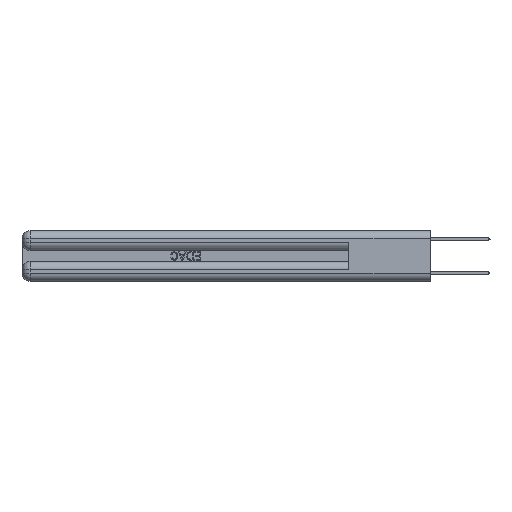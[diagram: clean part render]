
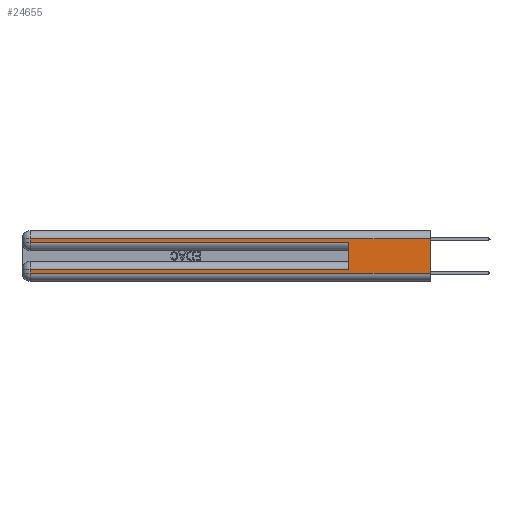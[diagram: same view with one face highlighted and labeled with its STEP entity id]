
A CAD part, left-side view. The second image highlights one B-rep face of the part: STEP entity #24655.
In plain terms, the highlighted planar face has unit normal (-1, 0, 0).
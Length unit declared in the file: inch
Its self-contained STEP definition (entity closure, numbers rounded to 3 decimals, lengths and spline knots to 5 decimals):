
#192 = DIRECTION ( 'NONE',  ( 0., 0., -1. ) ) ;
#230 = VERTEX_POINT ( 'NONE', #11451 ) ;
#247 = VERTEX_POINT ( 'NONE', #9179 ) ;
#296 = VECTOR ( 'NONE', #5717, 39.37008 ) ;
#312 = CARTESIAN_POINT ( 'NONE',  ( 0., 0.6, 0.285 ) ) ;
#361 = VERTEX_POINT ( 'NONE', #24869 ) ;
#596 = ORIENTED_EDGE ( 'NONE', *, *, #27372, .T. ) ;
#1087 = CARTESIAN_POINT ( 'NONE',  ( 0., 0.6, 0.145 ) ) ;
#1525 = CARTESIAN_POINT ( 'NONE',  ( 0., 2.94, 0.37 ) ) ;
#1733 = CARTESIAN_POINT ( 'NONE',  ( 0., 0., 0.06 ) ) ;
#2167 = CARTESIAN_POINT ( 'NONE',  ( 0., 2.94, 0.06 ) ) ;
#3639 = EDGE_CURVE ( 'NONE', #230, #12751, #26774, .T. ) ;
#4480 = PLANE ( 'NONE',  #22004 ) ;
#5116 = VERTEX_POINT ( 'NONE', #23936 ) ;
#5717 = DIRECTION ( 'NONE',  ( 0., 1., 0. ) ) ;
#5820 = LINE ( 'NONE', #12741, #21688 ) ;
#7189 = EDGE_CURVE ( 'NONE', #23041, #247, #27964, .T. ) ;
#8208 = DIRECTION ( 'NONE',  ( 0., -1., 0. ) ) ;
#8730 = CARTESIAN_POINT ( 'NONE',  ( 0., 2.94, 0.37 ) ) ;
#9179 = CARTESIAN_POINT ( 'NONE',  ( 0., 0., 0.06 ) ) ;
#9266 = CARTESIAN_POINT ( 'NONE',  ( 0., 0., 0.31 ) ) ;
#9878 = CARTESIAN_POINT ( 'NONE',  ( 0., 0., 0.085 ) ) ;
#10359 = ORIENTED_EDGE ( 'NONE', *, *, #12345, .F. ) ;
#11451 = CARTESIAN_POINT ( 'NONE',  ( 0., 0.6, 0.085 ) ) ;
#11720 = VERTEX_POINT ( 'NONE', #25460 ) ;
#11728 = LINE ( 'NONE', #9266, #27562 ) ;
#12126 = ORIENTED_EDGE ( 'NONE', *, *, #3639, .F. ) ;
#12345 = EDGE_CURVE ( 'NONE', #15269, #247, #18260, .T. ) ;
#12392 = DIRECTION ( 'NONE',  ( 0., 0., -1. ) ) ;
#12741 = CARTESIAN_POINT ( 'NONE',  ( 0., 0., 0.285 ) ) ;
#12751 = VERTEX_POINT ( 'NONE', #312 ) ;
#14152 = VECTOR ( 'NONE', #12392, 39.37008 ) ;
#14331 = VECTOR ( 'NONE', #18559, 39.37008 ) ;
#14810 = LINE ( 'NONE', #8730, #25882 ) ;
#14822 = DIRECTION ( 'NONE',  ( 0., 0., -1. ) ) ;
#15123 = DIRECTION ( 'NONE',  ( 0., 1., 0. ) ) ;
#15269 = VERTEX_POINT ( 'NONE', #18338 ) ;
#15449 = ORIENTED_EDGE ( 'NONE', *, *, #24988, .T. ) ;
#17200 = FACE_OUTER_BOUND ( 'NONE', #26297, .T. ) ;
#17418 = DIRECTION ( 'NONE',  ( 1., 0., 0. ) ) ;
#17863 = LINE ( 'NONE', #1525, #14152 ) ;
#17918 = ORIENTED_EDGE ( 'NONE', *, *, #7189, .T. ) ;
#18260 = LINE ( 'NONE', #27507, #23291 ) ;
#18338 = CARTESIAN_POINT ( 'NONE',  ( 0., 0., 0.31 ) ) ;
#18559 = DIRECTION ( 'NONE',  ( 0., 0., 1. ) ) ;
#18565 = LINE ( 'NONE', #9878, #296 ) ;
#18575 = EDGE_CURVE ( 'NONE', #11720, #12751, #5820, .T. ) ;
#20685 = DIRECTION ( 'NONE',  ( 0., -1., 0. ) ) ;
#21052 = ORIENTED_EDGE ( 'NONE', *, *, #18575, .T. ) ;
#21360 = ORIENTED_EDGE ( 'NONE', *, *, #24446, .T. ) ;
#21585 = ORIENTED_EDGE ( 'NONE', *, *, #27872, .T. ) ;
#21651 = DIRECTION ( 'NONE',  ( 0., 0., -1. ) ) ;
#21688 = VECTOR ( 'NONE', #8208, 39.37008 ) ;
#22004 = AXIS2_PLACEMENT_3D ( 'NONE', #23604, #17418, #192 ) ;
#23041 = VERTEX_POINT ( 'NONE', #2167 ) ;
#23291 = VECTOR ( 'NONE', #14822, 39.37008 ) ;
#23604 = CARTESIAN_POINT ( 'NONE',  ( 0., 0., 0.37 ) ) ;
#23936 = CARTESIAN_POINT ( 'NONE',  ( 0., 2.94, 0.085 ) ) ;
#24446 = EDGE_CURVE ( 'NONE', #230, #5116, #18565, .T. ) ;
#24655 = ADVANCED_FACE ( 'NONE', ( #17200 ), #4480, .F. ) ;
#24869 = CARTESIAN_POINT ( 'NONE',  ( 0., 2.94, 0.31 ) ) ;
#24988 = EDGE_CURVE ( 'NONE', #361, #11720, #17863, .T. ) ;
#25460 = CARTESIAN_POINT ( 'NONE',  ( 0., 2.94, 0.285 ) ) ;
#25882 = VECTOR ( 'NONE', #21651, 39.37008 ) ;
#26297 = EDGE_LOOP ( 'NONE', ( #10359, #21585, #15449, #21052, #12126, #21360, #596, #17918 ) ) ;
#26774 = LINE ( 'NONE', #1087, #14331 ) ;
#26927 = VECTOR ( 'NONE', #20685, 39.37008 ) ;
#27372 = EDGE_CURVE ( 'NONE', #5116, #23041, #14810, .T. ) ;
#27507 = CARTESIAN_POINT ( 'NONE',  ( 0., 0., 0.37 ) ) ;
#27562 = VECTOR ( 'NONE', #15123, 39.37008 ) ;
#27872 = EDGE_CURVE ( 'NONE', #15269, #361, #11728, .T. ) ;
#27964 = LINE ( 'NONE', #1733, #26927 ) ;
